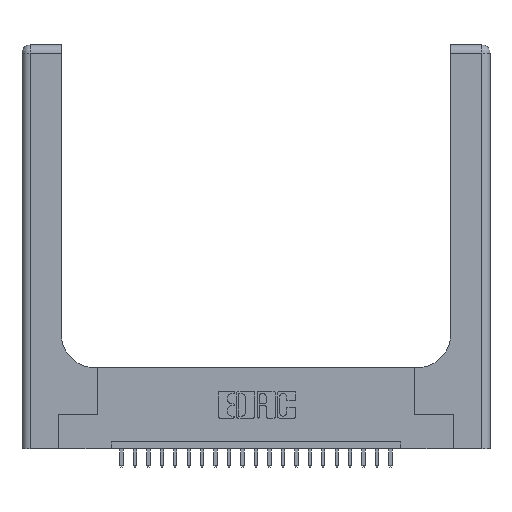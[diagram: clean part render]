
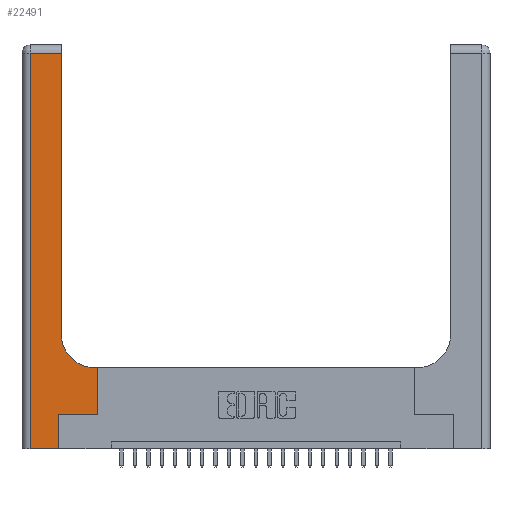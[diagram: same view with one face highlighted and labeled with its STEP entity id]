
A CAD part, top view. The second image highlights one B-rep face of the part: STEP entity #22491.
In plain terms, the highlighted planar face has unit normal (0, 0, 1).
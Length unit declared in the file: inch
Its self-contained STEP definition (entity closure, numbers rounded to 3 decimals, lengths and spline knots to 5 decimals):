
#237 = DIRECTION ( 'NONE',  ( 0., 0., -1. ) ) ;
#249 = VECTOR ( 'NONE', #21086, 39.37008 ) ;
#460 = CARTESIAN_POINT ( 'NONE',  ( 0.5415, 0.85, 0.37 ) ) ;
#937 = CARTESIAN_POINT ( 'NONE',  ( 0.269, 0., 0.37 ) ) ;
#1205 = VERTEX_POINT ( 'NONE', #1435 ) ;
#1435 = CARTESIAN_POINT ( 'NONE',  ( 0.5415, 0.6, 0.37 ) ) ;
#1451 = EDGE_CURVE ( 'NONE', #15579, #4908, #5061, .T. ) ;
#2305 = LINE ( 'NONE', #20092, #9176 ) ;
#2405 = LINE ( 'NONE', #9680, #4683 ) ;
#2425 = CARTESIAN_POINT ( 'NONE',  ( 0.269, 0.25, 0.37 ) ) ;
#2671 = ORIENTED_EDGE ( 'NONE', *, *, #5005, .T. ) ;
#3357 = VECTOR ( 'NONE', #23835, 39.37008 ) ;
#3466 = VERTEX_POINT ( 'NONE', #12393 ) ;
#3676 = LINE ( 'NONE', #8852, #7980 ) ;
#3909 = EDGE_CURVE ( 'NONE', #3466, #18310, #19099, .T. ) ;
#4683 = VECTOR ( 'NONE', #20405, 39.37008 ) ;
#4908 = VERTEX_POINT ( 'NONE', #937 ) ;
#5005 = EDGE_CURVE ( 'NONE', #4908, #19906, #5100, .T. ) ;
#5061 = LINE ( 'NONE', #7133, #3357 ) ;
#5100 = LINE ( 'NONE', #5543, #249 ) ;
#5220 = DIRECTION ( 'NONE',  ( 0., 1., 0. ) ) ;
#5411 = VERTEX_POINT ( 'NONE', #17851 ) ;
#5543 = CARTESIAN_POINT ( 'NONE',  ( 0.269, 0., 0.37 ) ) ;
#5614 = PLANE ( 'NONE',  #11073 ) ;
#5923 = VERTEX_POINT ( 'NONE', #23774 ) ;
#6195 = EDGE_CURVE ( 'NONE', #19906, #5923, #19718, .T. ) ;
#7133 = CARTESIAN_POINT ( 'NONE',  ( 0., 0., 0.37 ) ) ;
#7539 = EDGE_CURVE ( 'NONE', #21129, #15579, #2405, .T. ) ;
#7980 = VECTOR ( 'NONE', #12602, 39.37008 ) ;
#8825 = CIRCLE ( 'NONE', #19987, 0.25 ) ;
#8852 = CARTESIAN_POINT ( 'NONE',  ( 0.5585, 0.25, 0.37 ) ) ;
#9176 = VECTOR ( 'NONE', #12820, 39.37008 ) ;
#9271 = EDGE_CURVE ( 'NONE', #1205, #3466, #8825, .T. ) ;
#9591 = ORIENTED_EDGE ( 'NONE', *, *, #6195, .T. ) ;
#9680 = CARTESIAN_POINT ( 'NONE',  ( 0.06, 3., 0.37 ) ) ;
#10062 = ORIENTED_EDGE ( 'NONE', *, *, #16807, .T. ) ;
#10270 = DIRECTION ( 'NONE',  ( 1., 0., 0. ) ) ;
#10289 = ORIENTED_EDGE ( 'NONE', *, *, #14981, .T. ) ;
#11073 = AXIS2_PLACEMENT_3D ( 'NONE', #11236, #16480, #22113 ) ;
#11236 = CARTESIAN_POINT ( 'NONE',  ( 0., 3., 0.37 ) ) ;
#11380 = ORIENTED_EDGE ( 'NONE', *, *, #9271, .T. ) ;
#11506 = EDGE_LOOP ( 'NONE', ( #13231, #10289, #14003, #13312, #2671, #9591, #19785, #10062, #11380 ) ) ;
#12393 = CARTESIAN_POINT ( 'NONE',  ( 0.2915, 0.85, 0.37 ) ) ;
#12602 = DIRECTION ( 'NONE',  ( 0., 1., 0. ) ) ;
#12820 = DIRECTION ( 'NONE',  ( -1., 0., 0. ) ) ;
#12985 = VECTOR ( 'NONE', #18086, 39.37008 ) ;
#13082 = VECTOR ( 'NONE', #10270, 39.37008 ) ;
#13231 = ORIENTED_EDGE ( 'NONE', *, *, #3909, .T. ) ;
#13312 = ORIENTED_EDGE ( 'NONE', *, *, #1451, .T. ) ;
#14003 = ORIENTED_EDGE ( 'NONE', *, *, #7539, .T. ) ;
#14086 = CARTESIAN_POINT ( 'NONE',  ( 0.2915, 3., 0.37 ) ) ;
#14981 = EDGE_CURVE ( 'NONE', #18310, #21129, #15584, .T. ) ;
#15344 = CARTESIAN_POINT ( 'NONE',  ( 0.2915, 2.94, 0.37 ) ) ;
#15579 = VERTEX_POINT ( 'NONE', #22372 ) ;
#15584 = LINE ( 'NONE', #23811, #12985 ) ;
#16480 = DIRECTION ( 'NONE',  ( 0., 0., -1. ) ) ;
#16807 = EDGE_CURVE ( 'NONE', #5411, #1205, #2305, .T. ) ;
#17851 = CARTESIAN_POINT ( 'NONE',  ( 0.5585, 0.6, 0.37 ) ) ;
#17995 = EDGE_CURVE ( 'NONE', #5923, #5411, #3676, .T. ) ;
#18086 = DIRECTION ( 'NONE',  ( -1., 0., 0. ) ) ;
#18310 = VERTEX_POINT ( 'NONE', #15344 ) ;
#19099 = LINE ( 'NONE', #14086, #22259 ) ;
#19196 = CARTESIAN_POINT ( 'NONE',  ( 0.06, 2.94, 0.37 ) ) ;
#19718 = LINE ( 'NONE', #2425, #13082 ) ;
#19785 = ORIENTED_EDGE ( 'NONE', *, *, #17995, .T. ) ;
#19906 = VERTEX_POINT ( 'NONE', #20451 ) ;
#19987 = AXIS2_PLACEMENT_3D ( 'NONE', #460, #237, #22407 ) ;
#20092 = CARTESIAN_POINT ( 'NONE',  ( 0.2915, 0.6, 0.37 ) ) ;
#20405 = DIRECTION ( 'NONE',  ( 0., -1., 0. ) ) ;
#20451 = CARTESIAN_POINT ( 'NONE',  ( 0.269, 0.25, 0.37 ) ) ;
#21086 = DIRECTION ( 'NONE',  ( 0., 1., 0. ) ) ;
#21129 = VERTEX_POINT ( 'NONE', #19196 ) ;
#22113 = DIRECTION ( 'NONE',  ( -1., 0., 0. ) ) ;
#22259 = VECTOR ( 'NONE', #5220, 39.37008 ) ;
#22372 = CARTESIAN_POINT ( 'NONE',  ( 0.06, 0., 0.37 ) ) ;
#22407 = DIRECTION ( 'NONE',  ( 1., 0., 0. ) ) ;
#22491 = ADVANCED_FACE ( 'NONE', ( #23857 ), #5614, .F. ) ;
#23774 = CARTESIAN_POINT ( 'NONE',  ( 0.5585, 0.25, 0.37 ) ) ;
#23811 = CARTESIAN_POINT ( 'NONE',  ( 0., 2.94, 0.37 ) ) ;
#23835 = DIRECTION ( 'NONE',  ( 1., 0., 0. ) ) ;
#23857 = FACE_OUTER_BOUND ( 'NONE', #11506, .T. ) ;
